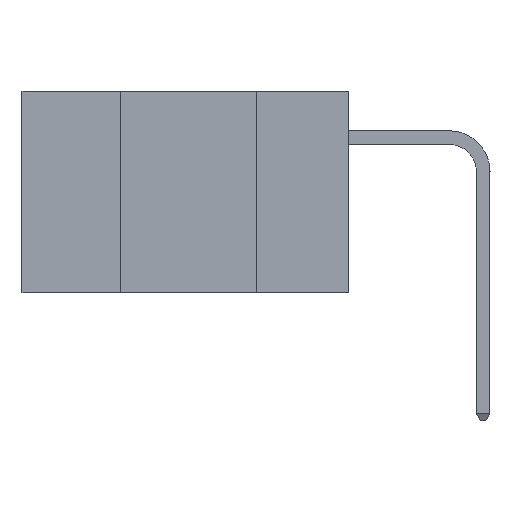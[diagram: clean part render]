
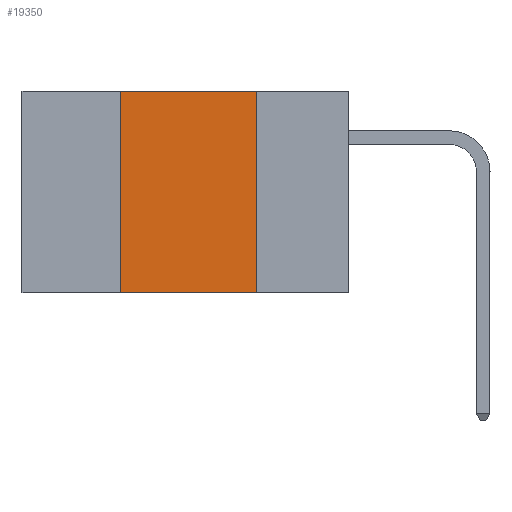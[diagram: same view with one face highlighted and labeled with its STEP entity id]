
A CAD part, left-side view. The second image highlights one B-rep face of the part: STEP entity #19350.
In plain terms, the highlighted planar face has unit normal (-1, 0, 0).
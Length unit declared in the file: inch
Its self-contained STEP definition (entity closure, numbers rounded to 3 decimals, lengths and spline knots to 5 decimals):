
#4 = LINE ( 'NONE', #8804, #23906 ) ;
#206 = EDGE_CURVE ( 'NONE', #27097, #24523, #5573, .T. ) ;
#573 = FACE_OUTER_BOUND ( 'NONE', #23297, .T. ) ;
#946 = EDGE_CURVE ( 'NONE', #17411, #23355, #4, .T. ) ;
#2301 = CARTESIAN_POINT ( 'NONE',  ( 0., 0.17, 0. ) ) ;
#2544 = EDGE_CURVE ( 'NONE', #23355, #24523, #18543, .T. ) ;
#3239 = DIRECTION ( 'NONE',  ( 0., 0., -1. ) ) ;
#3500 = ORIENTED_EDGE ( 'NONE', *, *, #946, .F. ) ;
#3786 = CARTESIAN_POINT ( 'NONE',  ( 0., 0.42, -0.37 ) ) ;
#4975 = EDGE_CURVE ( 'NONE', #27097, #17411, #11905, .T. ) ;
#5544 = VECTOR ( 'NONE', #3239, 39.37008 ) ;
#5573 = LINE ( 'NONE', #11922, #23888 ) ;
#7422 = CARTESIAN_POINT ( 'NONE',  ( 0., 0.42, 0. ) ) ;
#8804 = CARTESIAN_POINT ( 'NONE',  ( 0., 0.6, 0. ) ) ;
#11270 = ORIENTED_EDGE ( 'NONE', *, *, #4975, .F. ) ;
#11301 = AXIS2_PLACEMENT_3D ( 'NONE', #16313, #20660, #18480 ) ;
#11905 = LINE ( 'NONE', #7422, #17363 ) ;
#11922 = CARTESIAN_POINT ( 'NONE',  ( 0., 0.6, -0.37 ) ) ;
#13799 = ORIENTED_EDGE ( 'NONE', *, *, #2544, .F. ) ;
#13949 = DIRECTION ( 'NONE',  ( 0., -1., 0. ) ) ;
#14182 = CARTESIAN_POINT ( 'NONE',  ( 0., 0.42, 0. ) ) ;
#16313 = CARTESIAN_POINT ( 'NONE',  ( 0., 0.6, 0. ) ) ;
#17363 = VECTOR ( 'NONE', #18557, 39.37008 ) ;
#17411 = VERTEX_POINT ( 'NONE', #14182 ) ;
#18480 = DIRECTION ( 'NONE',  ( 0., 0., -1. ) ) ;
#18543 = LINE ( 'NONE', #23028, #5544 ) ;
#18557 = DIRECTION ( 'NONE',  ( 0., 0., 1. ) ) ;
#19350 = ADVANCED_FACE ( 'NONE', ( #573 ), #22524, .F. ) ;
#20660 = DIRECTION ( 'NONE',  ( 1., 0., 0. ) ) ;
#22524 = PLANE ( 'NONE',  #11301 ) ;
#22911 = DIRECTION ( 'NONE',  ( 0., -1., 0. ) ) ;
#23028 = CARTESIAN_POINT ( 'NONE',  ( 0., 0.17, 0. ) ) ;
#23297 = EDGE_LOOP ( 'NONE', ( #13799, #3500, #11270, #25311 ) ) ;
#23355 = VERTEX_POINT ( 'NONE', #2301 ) ;
#23888 = VECTOR ( 'NONE', #22911, 39.37008 ) ;
#23906 = VECTOR ( 'NONE', #13949, 39.37008 ) ;
#24523 = VERTEX_POINT ( 'NONE', #26001 ) ;
#25311 = ORIENTED_EDGE ( 'NONE', *, *, #206, .T. ) ;
#26001 = CARTESIAN_POINT ( 'NONE',  ( 0., 0.17, -0.37 ) ) ;
#27097 = VERTEX_POINT ( 'NONE', #3786 ) ;
